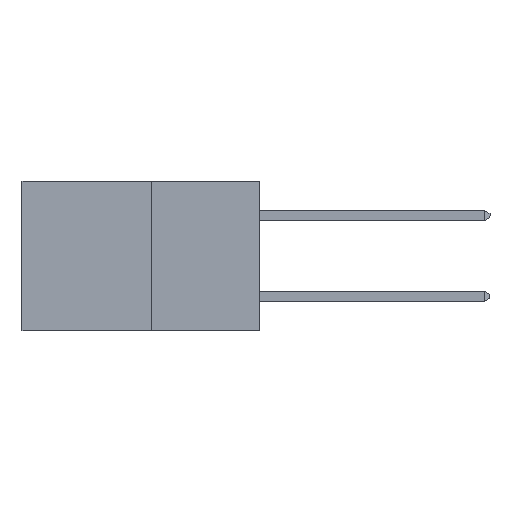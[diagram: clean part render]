
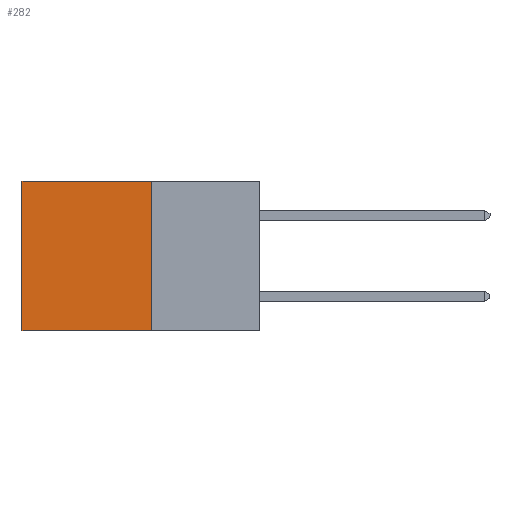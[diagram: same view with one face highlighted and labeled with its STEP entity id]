
A CAD part, left-side view. The second image highlights one B-rep face of the part: STEP entity #282.
In plain terms, the highlighted planar face has unit normal (-1, 0, 0).
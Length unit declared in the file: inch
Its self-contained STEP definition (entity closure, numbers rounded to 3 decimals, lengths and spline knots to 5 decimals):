
#51 = CARTESIAN_POINT ( 'NONE',  ( 0.277, 0.59, 0. ) ) ;
#282 = ADVANCED_FACE ( 'NONE', ( #2339 ), #6060, .F. ) ;
#415 = EDGE_CURVE ( 'NONE', #737, #8195, #8116, .T. ) ;
#737 = VERTEX_POINT ( 'NONE', #1690 ) ;
#854 = VECTOR ( 'NONE', #2074, 39.37008 ) ;
#1151 = ORIENTED_EDGE ( 'NONE', *, *, #3421, .T. ) ;
#1368 = VERTEX_POINT ( 'NONE', #51 ) ;
#1488 = LINE ( 'NONE', #2746, #8162 ) ;
#1563 = DIRECTION ( 'NONE',  ( 1., 0., 0. ) ) ;
#1690 = CARTESIAN_POINT ( 'NONE',  ( 0.277, 0.27, 0. ) ) ;
#2074 = DIRECTION ( 'NONE',  ( 0., 0., -1. ) ) ;
#2130 = CARTESIAN_POINT ( 'NONE',  ( 0.277, 0.27, -0.37 ) ) ;
#2220 = CARTESIAN_POINT ( 'NONE',  ( 0.277, 0.59, -0.37 ) ) ;
#2339 = FACE_OUTER_BOUND ( 'NONE', #5944, .T. ) ;
#2373 = ORIENTED_EDGE ( 'NONE', *, *, #415, .F. ) ;
#2409 = CARTESIAN_POINT ( 'NONE',  ( 0.277, 0.59, -0.37 ) ) ;
#2746 = CARTESIAN_POINT ( 'NONE',  ( 0.277, 0.27, 0. ) ) ;
#3421 = EDGE_CURVE ( 'NONE', #737, #1368, #1488, .T. ) ;
#3508 = EDGE_CURVE ( 'NONE', #1368, #6736, #4248, .T. ) ;
#3659 = EDGE_CURVE ( 'NONE', #8195, #6736, #4919, .T. ) ;
#3854 = VECTOR ( 'NONE', #6164, 39.37008 ) ;
#4248 = LINE ( 'NONE', #2220, #854 ) ;
#4333 = CARTESIAN_POINT ( 'NONE',  ( 0.277, 0.27, -0.37 ) ) ;
#4667 = CARTESIAN_POINT ( 'NONE',  ( 0.277, 0.27, -0.37 ) ) ;
#4919 = LINE ( 'NONE', #6145, #3854 ) ;
#5712 = DIRECTION ( 'NONE',  ( 0., 0., -1. ) ) ;
#5944 = EDGE_LOOP ( 'NONE', ( #6249, #7312, #2373, #1151 ) ) ;
#6060 = PLANE ( 'NONE',  #6717 ) ;
#6145 = CARTESIAN_POINT ( 'NONE',  ( 0.277, 0.27, -0.37 ) ) ;
#6164 = DIRECTION ( 'NONE',  ( 0., 1., 0. ) ) ;
#6249 = ORIENTED_EDGE ( 'NONE', *, *, #3508, .T. ) ;
#6451 = DIRECTION ( 'NONE',  ( 0., 1., 0. ) ) ;
#6510 = VECTOR ( 'NONE', #7991, 39.37008 ) ;
#6717 = AXIS2_PLACEMENT_3D ( 'NONE', #4667, #1563, #5712 ) ;
#6736 = VERTEX_POINT ( 'NONE', #2409 ) ;
#7312 = ORIENTED_EDGE ( 'NONE', *, *, #3659, .F. ) ;
#7991 = DIRECTION ( 'NONE',  ( 0., 0., -1. ) ) ;
#8116 = LINE ( 'NONE', #4333, #6510 ) ;
#8162 = VECTOR ( 'NONE', #6451, 39.37008 ) ;
#8195 = VERTEX_POINT ( 'NONE', #2130 ) ;
